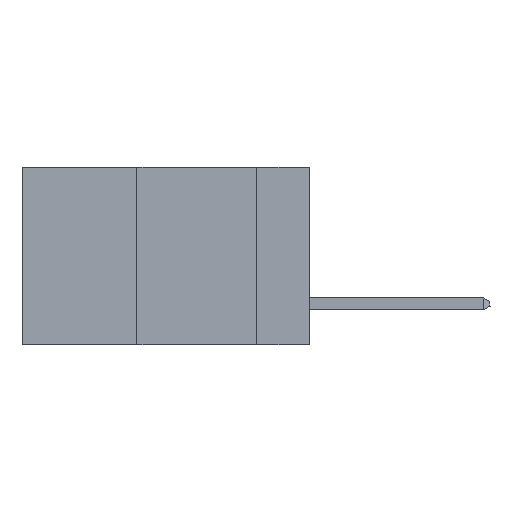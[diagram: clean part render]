
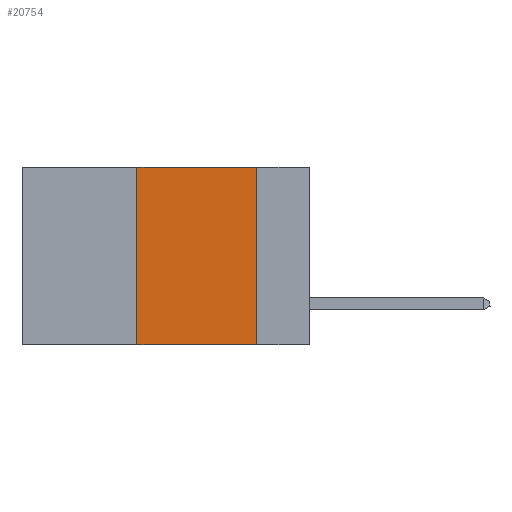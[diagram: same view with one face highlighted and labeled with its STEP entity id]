
A CAD part, left-side view. The second image highlights one B-rep face of the part: STEP entity #20754.
In plain terms, the highlighted planar face has unit normal (-1, 0, 0).
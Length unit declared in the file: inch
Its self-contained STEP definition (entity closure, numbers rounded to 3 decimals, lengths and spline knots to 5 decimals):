
#373 = ORIENTED_EDGE ( 'NONE', *, *, #25514, .F. ) ;
#546 = CARTESIAN_POINT ( 'NONE',  ( 0., 0.11, 0. ) ) ;
#1263 = LINE ( 'NONE', #16667, #19251 ) ;
#3931 = EDGE_CURVE ( 'NONE', #27351, #27976, #27386, .T. ) ;
#7370 = DIRECTION ( 'NONE',  ( 0., 0., -1. ) ) ;
#7971 = VECTOR ( 'NONE', #13812, 39.37008 ) ;
#9528 = VECTOR ( 'NONE', #19700, 39.37008 ) ;
#11638 = EDGE_LOOP ( 'NONE', ( #25897, #373, #13046, #24966 ) ) ;
#11805 = CARTESIAN_POINT ( 'NONE',  ( 0., 0.36, -0.37 ) ) ;
#12909 = CARTESIAN_POINT ( 'NONE',  ( 0., 0.6, 0. ) ) ;
#13046 = ORIENTED_EDGE ( 'NONE', *, *, #20817, .F. ) ;
#13439 = AXIS2_PLACEMENT_3D ( 'NONE', #14109, #18717, #7370 ) ;
#13698 = CARTESIAN_POINT ( 'NONE',  ( 0., 0.6, -0.37 ) ) ;
#13812 = DIRECTION ( 'NONE',  ( 0., 0., -1. ) ) ;
#14109 = CARTESIAN_POINT ( 'NONE',  ( 0., 0.6, 0. ) ) ;
#15079 = LINE ( 'NONE', #12909, #9528 ) ;
#15740 = VERTEX_POINT ( 'NONE', #11805 ) ;
#16189 = PLANE ( 'NONE',  #13439 ) ;
#16667 = CARTESIAN_POINT ( 'NONE',  ( 0., 0.36, 0. ) ) ;
#18717 = DIRECTION ( 'NONE',  ( 1., 0., 0. ) ) ;
#18990 = DIRECTION ( 'NONE',  ( 0., -1., 0. ) ) ;
#19251 = VECTOR ( 'NONE', #23258, 39.37008 ) ;
#19608 = CARTESIAN_POINT ( 'NONE',  ( 0., 0.36, 0. ) ) ;
#19700 = DIRECTION ( 'NONE',  ( 0., -1., 0. ) ) ;
#20239 = EDGE_CURVE ( 'NONE', #15740, #27976, #20296, .T. ) ;
#20296 = LINE ( 'NONE', #13698, #25483 ) ;
#20754 = ADVANCED_FACE ( 'NONE', ( #24060 ), #16189, .F. ) ;
#20817 = EDGE_CURVE ( 'NONE', #15740, #25586, #1263, .T. ) ;
#22072 = CARTESIAN_POINT ( 'NONE',  ( 0., 0.11, -0.37 ) ) ;
#23258 = DIRECTION ( 'NONE',  ( 0., 0., 1. ) ) ;
#24060 = FACE_OUTER_BOUND ( 'NONE', #11638, .T. ) ;
#24211 = CARTESIAN_POINT ( 'NONE',  ( 0., 0.11, 0. ) ) ;
#24966 = ORIENTED_EDGE ( 'NONE', *, *, #20239, .T. ) ;
#25483 = VECTOR ( 'NONE', #18990, 39.37008 ) ;
#25514 = EDGE_CURVE ( 'NONE', #25586, #27351, #15079, .T. ) ;
#25586 = VERTEX_POINT ( 'NONE', #19608 ) ;
#25897 = ORIENTED_EDGE ( 'NONE', *, *, #3931, .F. ) ;
#27351 = VERTEX_POINT ( 'NONE', #24211 ) ;
#27386 = LINE ( 'NONE', #546, #7971 ) ;
#27976 = VERTEX_POINT ( 'NONE', #22072 ) ;
